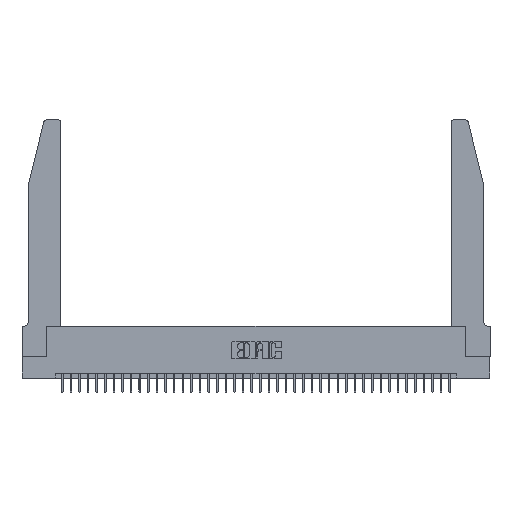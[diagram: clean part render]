
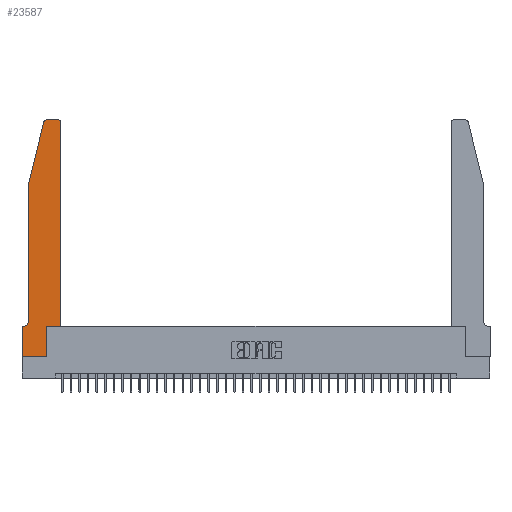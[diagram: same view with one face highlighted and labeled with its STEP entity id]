
A CAD part, top view. The second image highlights one B-rep face of the part: STEP entity #23587.
In plain terms, the highlighted planar face has unit normal (0, 0, 1).
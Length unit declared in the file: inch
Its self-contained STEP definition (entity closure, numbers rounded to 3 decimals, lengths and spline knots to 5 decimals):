
#181 = AXIS2_PLACEMENT_3D ( 'NONE', #430, #22405, #3638 ) ;
#188 = CARTESIAN_POINT ( 'NONE',  ( 0.4205, 2.75, 0.37 ) ) ;
#430 = CARTESIAN_POINT ( 'NONE',  ( 0.4205, 2.72, 0.37 ) ) ;
#515 = LINE ( 'NONE', #36688, #7957 ) ;
#664 = DIRECTION ( 'NONE',  ( 0., -1., 0. ) ) ;
#669 = LINE ( 'NONE', #28337, #33890 ) ;
#916 = LINE ( 'NONE', #25548, #16746 ) ;
#1992 = CARTESIAN_POINT ( 'NONE',  ( 0.2865, 0., 0.37 ) ) ;
#2192 = VERTEX_POINT ( 'NONE', #15181 ) ;
#2256 = EDGE_CURVE ( 'NONE', #9530, #27130, #28382, .T. ) ;
#2259 = VERTEX_POINT ( 'NONE', #24774 ) ;
#2435 = CARTESIAN_POINT ( 'NONE',  ( 0.0755, 0.35, 0.37 ) ) ;
#2694 = AXIS2_PLACEMENT_3D ( 'NONE', #9208, #30940, #12394 ) ;
#2830 = VECTOR ( 'NONE', #21733, 39.37008 ) ;
#3233 = CARTESIAN_POINT ( 'NONE',  ( 0.4505, 2.72, 0.37 ) ) ;
#3482 = DIRECTION ( 'NONE',  ( 0., 0., 1. ) ) ;
#3638 = DIRECTION ( 'NONE',  ( 1., 0., 0. ) ) ;
#3678 = LINE ( 'NONE', #16271, #36784 ) ;
#3720 = DIRECTION ( 'NONE',  ( 1., 0., 0. ) ) ;
#4019 = CARTESIAN_POINT ( 'NONE',  ( 0., 0., 0.37 ) ) ;
#4391 = ORIENTED_EDGE ( 'NONE', *, *, #34775, .T. ) ;
#5220 = VERTEX_POINT ( 'NONE', #188 ) ;
#5936 = CIRCLE ( 'NONE', #181, 0.03 ) ;
#6938 = CARTESIAN_POINT ( 'NONE',  ( 0.0055, 0.35, 0.37 ) ) ;
#6953 = DIRECTION ( 'NONE',  ( 0., -1., 0. ) ) ;
#7641 = EDGE_CURVE ( 'NONE', #14477, #18680, #669, .T. ) ;
#7957 = VECTOR ( 'NONE', #24422, 39.37008 ) ;
#8079 = VERTEX_POINT ( 'NONE', #18337 ) ;
#8516 = CARTESIAN_POINT ( 'NONE',  ( 0.4505, 0.35, 0.37 ) ) ;
#8523 = VERTEX_POINT ( 'NONE', #17387 ) ;
#9042 = ORIENTED_EDGE ( 'NONE', *, *, #20499, .T. ) ;
#9208 = CARTESIAN_POINT ( 'NONE',  ( 0.0055, 0.42, 0.37 ) ) ;
#9290 = DIRECTION ( 'NONE',  ( 0., 1., 0. ) ) ;
#9530 = VERTEX_POINT ( 'NONE', #13910 ) ;
#10097 = EDGE_CURVE ( 'NONE', #38165, #5220, #5936, .T. ) ;
#10503 = FACE_OUTER_BOUND ( 'NONE', #16645, .T. ) ;
#11520 = DIRECTION ( 'NONE',  ( 0., 0., 1. ) ) ;
#12394 = DIRECTION ( 'NONE',  ( -1., 0., 0. ) ) ;
#13213 = VECTOR ( 'NONE', #664, 39.37008 ) ;
#13910 = CARTESIAN_POINT ( 'NONE',  ( 0.0755, 0.42, 0.37 ) ) ;
#14217 = ORIENTED_EDGE ( 'NONE', *, *, #39906, .T. ) ;
#14477 = VERTEX_POINT ( 'NONE', #1992 ) ;
#15181 = CARTESIAN_POINT ( 'NONE',  ( 0., 0., 0.37 ) ) ;
#15774 = LINE ( 'NONE', #2435, #23047 ) ;
#16032 = CARTESIAN_POINT ( 'NONE',  ( 0., 0.35, 0.37 ) ) ;
#16271 = CARTESIAN_POINT ( 'NONE',  ( 0.4505, 0.35, 0.37 ) ) ;
#16440 = ORIENTED_EDGE ( 'NONE', *, *, #2256, .T. ) ;
#16512 = EDGE_CURVE ( 'NONE', #5220, #16608, #27765, .T. ) ;
#16608 = VERTEX_POINT ( 'NONE', #22154 ) ;
#16645 = EDGE_LOOP ( 'NONE', ( #27781, #14217, #25203, #4391, #16440, #35358, #38488, #9042, #34174, #30084, #16715, #30254 ) ) ;
#16715 = ORIENTED_EDGE ( 'NONE', *, *, #37379, .T. ) ;
#16746 = VECTOR ( 'NONE', #6953, 39.37008 ) ;
#16904 = VECTOR ( 'NONE', #24230, 39.37008 ) ;
#17387 = CARTESIAN_POINT ( 'NONE',  ( 0., 0.35, 0.37 ) ) ;
#18337 = CARTESIAN_POINT ( 'NONE',  ( 0.0755, 2., 0.37 ) ) ;
#18680 = VERTEX_POINT ( 'NONE', #21838 ) ;
#18782 = AXIS2_PLACEMENT_3D ( 'NONE', #16032, #3482, #25374 ) ;
#19489 = AXIS2_PLACEMENT_3D ( 'NONE', #30083, #11520, #33208 ) ;
#20499 = EDGE_CURVE ( 'NONE', #2192, #14477, #23665, .T. ) ;
#21733 = DIRECTION ( 'NONE',  ( -1., 0., 0. ) ) ;
#21838 = CARTESIAN_POINT ( 'NONE',  ( 0.2865, 0.35, 0.37 ) ) ;
#22154 = CARTESIAN_POINT ( 'NONE',  ( 0.284, 2.75, 0.37 ) ) ;
#22257 = PLANE ( 'NONE',  #18782 ) ;
#22405 = DIRECTION ( 'NONE',  ( 0., 0., 1. ) ) ;
#22658 = CARTESIAN_POINT ( 'NONE',  ( 0.0755, 2., 0.37 ) ) ;
#23047 = VECTOR ( 'NONE', #27464, 39.37008 ) ;
#23587 = ADVANCED_FACE ( 'NONE', ( #10503 ), #22257, .T. ) ;
#23665 = LINE ( 'NONE', #4019, #30859 ) ;
#24230 = DIRECTION ( 'NONE',  ( 0., 1., 0. ) ) ;
#24422 = DIRECTION ( 'NONE',  ( -0.239, -0.971, 0. ) ) ;
#24774 = CARTESIAN_POINT ( 'NONE',  ( 0.4505, 0.35, 0.37 ) ) ;
#25203 = ORIENTED_EDGE ( 'NONE', *, *, #29694, .T. ) ;
#25374 = DIRECTION ( 'NONE',  ( 1., 0., 0. ) ) ;
#25548 = CARTESIAN_POINT ( 'NONE',  ( 0., 0., 0.37 ) ) ;
#25891 = DIRECTION ( 'NONE',  ( 1., 0., 0. ) ) ;
#26240 = EDGE_CURVE ( 'NONE', #27130, #8523, #15774, .T. ) ;
#27130 = VERTEX_POINT ( 'NONE', #6938 ) ;
#27260 = VERTEX_POINT ( 'NONE', #32490 ) ;
#27464 = DIRECTION ( 'NONE',  ( -1., 0., 0. ) ) ;
#27765 = LINE ( 'NONE', #27831, #2830 ) ;
#27781 = ORIENTED_EDGE ( 'NONE', *, *, #16512, .T. ) ;
#27783 = EDGE_CURVE ( 'NONE', #18680, #2259, #3678, .T. ) ;
#27831 = CARTESIAN_POINT ( 'NONE',  ( 0.2605, 2.75, 0.37 ) ) ;
#28337 = CARTESIAN_POINT ( 'NONE',  ( 0.2865, 0.35, 0.37 ) ) ;
#28382 = CIRCLE ( 'NONE', #2694, 0.07 ) ;
#29694 = EDGE_CURVE ( 'NONE', #27260, #8079, #515, .T. ) ;
#30083 = CARTESIAN_POINT ( 'NONE',  ( 0.284, 2.72, 0.37 ) ) ;
#30084 = ORIENTED_EDGE ( 'NONE', *, *, #27783, .T. ) ;
#30254 = ORIENTED_EDGE ( 'NONE', *, *, #10097, .T. ) ;
#30859 = VECTOR ( 'NONE', #25891, 39.37008 ) ;
#30940 = DIRECTION ( 'NONE',  ( 0., 0., -1. ) ) ;
#31268 = EDGE_CURVE ( 'NONE', #8523, #2192, #916, .T. ) ;
#32490 = CARTESIAN_POINT ( 'NONE',  ( 0.25487, 2.72718, 0.37 ) ) ;
#33208 = DIRECTION ( 'NONE',  ( 1., 0., 0. ) ) ;
#33303 = LINE ( 'NONE', #8516, #16904 ) ;
#33890 = VECTOR ( 'NONE', #9290, 39.37008 ) ;
#34174 = ORIENTED_EDGE ( 'NONE', *, *, #7641, .T. ) ;
#34307 = CIRCLE ( 'NONE', #19489, 0.03 ) ;
#34775 = EDGE_CURVE ( 'NONE', #8079, #9530, #35963, .T. ) ;
#35358 = ORIENTED_EDGE ( 'NONE', *, *, #26240, .T. ) ;
#35963 = LINE ( 'NONE', #22658, #13213 ) ;
#36688 = CARTESIAN_POINT ( 'NONE',  ( 0.0755, 2., 0.37 ) ) ;
#36784 = VECTOR ( 'NONE', #3720, 39.37008 ) ;
#37379 = EDGE_CURVE ( 'NONE', #2259, #38165, #33303, .T. ) ;
#38165 = VERTEX_POINT ( 'NONE', #3233 ) ;
#38488 = ORIENTED_EDGE ( 'NONE', *, *, #31268, .T. ) ;
#39906 = EDGE_CURVE ( 'NONE', #16608, #27260, #34307, .T. ) ;
